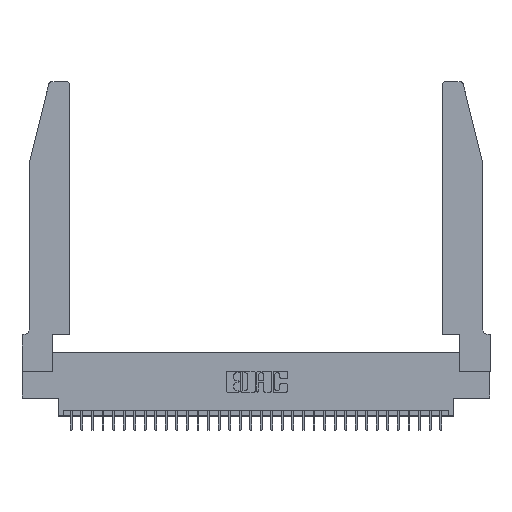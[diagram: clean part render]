
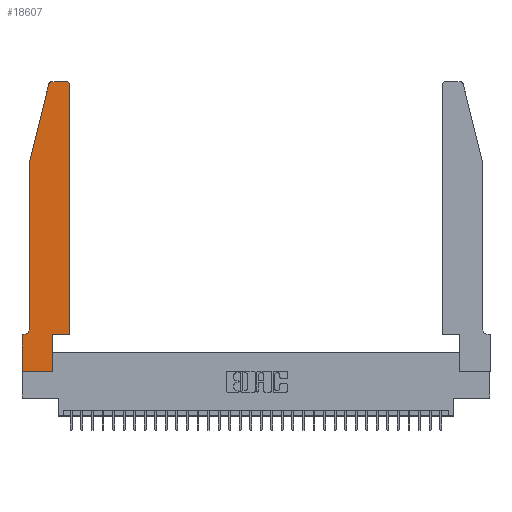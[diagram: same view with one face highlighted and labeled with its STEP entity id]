
A CAD part, top view. The second image highlights one B-rep face of the part: STEP entity #18607.
In plain terms, the highlighted planar face has unit normal (0, 0, 1).
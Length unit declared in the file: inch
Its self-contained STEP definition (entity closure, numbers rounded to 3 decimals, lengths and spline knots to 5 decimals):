
#76 = LINE ( 'NONE', #13323, #6920 ) ;
#954 = DIRECTION ( 'NONE',  ( 0., 1., 0. ) ) ;
#1054 = DIRECTION ( 'NONE',  ( 1., 0., 0. ) ) ;
#1309 = VERTEX_POINT ( 'NONE', #8028 ) ;
#1374 = EDGE_CURVE ( 'NONE', #4359, #28598, #26620, .T. ) ;
#1521 = CARTESIAN_POINT ( 'NONE',  ( 0., 0.35, 0.37 ) ) ;
#1557 = DIRECTION ( 'NONE',  ( 1., 0., 0. ) ) ;
#1675 = DIRECTION ( 'NONE',  ( 0., 0., 1. ) ) ;
#1846 = CARTESIAN_POINT ( 'NONE',  ( 0.2865, 0.35, 0.37 ) ) ;
#2091 = VERTEX_POINT ( 'NONE', #13837 ) ;
#2400 = VERTEX_POINT ( 'NONE', #10340 ) ;
#2531 = DIRECTION ( 'NONE',  ( 0., -1., 0. ) ) ;
#2763 = DIRECTION ( 'NONE',  ( 1., 0., 0. ) ) ;
#3043 = LINE ( 'NONE', #13527, #30806 ) ;
#3999 = AXIS2_PLACEMENT_3D ( 'NONE', #25015, #24501, #30032 ) ;
#4359 = VERTEX_POINT ( 'NONE', #29750 ) ;
#4598 = VECTOR ( 'NONE', #1557, 39.37008 ) ;
#4768 = CARTESIAN_POINT ( 'NONE',  ( 0.25487, 2.72718, 0.37 ) ) ;
#5093 = EDGE_CURVE ( 'NONE', #24850, #13024, #31501, .T. ) ;
#6107 = EDGE_CURVE ( 'NONE', #28598, #2400, #19819, .T. ) ;
#6110 = CARTESIAN_POINT ( 'NONE',  ( 0.2865, 0.35, 0.37 ) ) ;
#6686 = PLANE ( 'NONE',  #24319 ) ;
#6690 = EDGE_CURVE ( 'NONE', #1309, #9084, #20849, .T. ) ;
#6920 = VECTOR ( 'NONE', #24038, 39.37008 ) ;
#7410 = ORIENTED_EDGE ( 'NONE', *, *, #29518, .T. ) ;
#7415 = LINE ( 'NONE', #20180, #26383 ) ;
#7442 = EDGE_LOOP ( 'NONE', ( #7410, #22434, #31348, #13535, #31731, #28482, #27480, #15496, #32855, #11401, #15814, #26457 ) ) ;
#7660 = AXIS2_PLACEMENT_3D ( 'NONE', #24821, #19822, #1054 ) ;
#7762 = CARTESIAN_POINT ( 'NONE',  ( 0., 0., 0.37 ) ) ;
#8028 = CARTESIAN_POINT ( 'NONE',  ( 0., 0.35, 0.37 ) ) ;
#8782 = CARTESIAN_POINT ( 'NONE',  ( 0.4205, 2.72, 0.37 ) ) ;
#9084 = VERTEX_POINT ( 'NONE', #31562 ) ;
#9114 = DIRECTION ( 'NONE',  ( 0., 0., 1. ) ) ;
#9442 = DIRECTION ( 'NONE',  ( 1., 0., 0. ) ) ;
#9764 = EDGE_CURVE ( 'NONE', #28842, #2091, #22382, .T. ) ;
#10015 = LINE ( 'NONE', #20533, #29179 ) ;
#10340 = CARTESIAN_POINT ( 'NONE',  ( 0.4505, 0.35, 0.37 ) ) ;
#10406 = EDGE_CURVE ( 'NONE', #2400, #28842, #76, .T. ) ;
#11153 = VECTOR ( 'NONE', #21382, 39.37008 ) ;
#11401 = ORIENTED_EDGE ( 'NONE', *, *, #6107, .T. ) ;
#11603 = CARTESIAN_POINT ( 'NONE',  ( 0.0755, 0.42, 0.37 ) ) ;
#12979 = EDGE_CURVE ( 'NONE', #16748, #24606, #18082, .T. ) ;
#13024 = VERTEX_POINT ( 'NONE', #30683 ) ;
#13323 = CARTESIAN_POINT ( 'NONE',  ( 0.4505, 0.35, 0.37 ) ) ;
#13527 = CARTESIAN_POINT ( 'NONE',  ( 0.0755, 2., 0.37 ) ) ;
#13535 = ORIENTED_EDGE ( 'NONE', *, *, #13633, .T. ) ;
#13633 = EDGE_CURVE ( 'NONE', #23809, #24850, #3043, .T. ) ;
#13837 = CARTESIAN_POINT ( 'NONE',  ( 0.4205, 2.75, 0.37 ) ) ;
#15496 = ORIENTED_EDGE ( 'NONE', *, *, #16502, .T. ) ;
#15602 = VECTOR ( 'NONE', #23781, 39.37008 ) ;
#15814 = ORIENTED_EDGE ( 'NONE', *, *, #10406, .T. ) ;
#16332 = VECTOR ( 'NONE', #26514, 39.37008 ) ;
#16502 = EDGE_CURVE ( 'NONE', #9084, #4359, #10015, .T. ) ;
#16748 = VERTEX_POINT ( 'NONE', #29151 ) ;
#17347 = FACE_OUTER_BOUND ( 'NONE', #7442, .T. ) ;
#18082 = CIRCLE ( 'NONE', #7660, 0.03 ) ;
#18577 = LINE ( 'NONE', #23589, #16332 ) ;
#18607 = ADVANCED_FACE ( 'NONE', ( #17347 ), #6686, .T. ) ;
#19481 = CARTESIAN_POINT ( 'NONE',  ( 0.4505, 0.35, 0.37 ) ) ;
#19687 = EDGE_CURVE ( 'NONE', #13024, #1309, #28999, .T. ) ;
#19819 = LINE ( 'NONE', #19481, #4598 ) ;
#19822 = DIRECTION ( 'NONE',  ( 0., 0., 1. ) ) ;
#19948 = DIRECTION ( 'NONE',  ( 1., 0., 0. ) ) ;
#20180 = CARTESIAN_POINT ( 'NONE',  ( 0.2605, 2.75, 0.37 ) ) ;
#20533 = CARTESIAN_POINT ( 'NONE',  ( 0., 0., 0.37 ) ) ;
#20849 = LINE ( 'NONE', #7762, #15602 ) ;
#21382 = DIRECTION ( 'NONE',  ( -1., 0., 0. ) ) ;
#22382 = CIRCLE ( 'NONE', #25149, 0.03 ) ;
#22434 = ORIENTED_EDGE ( 'NONE', *, *, #12979, .T. ) ;
#23243 = DIRECTION ( 'NONE',  ( -1., 0., 0. ) ) ;
#23500 = CARTESIAN_POINT ( 'NONE',  ( 0.0755, 2., 0.37 ) ) ;
#23589 = CARTESIAN_POINT ( 'NONE',  ( 0.0755, 2., 0.37 ) ) ;
#23781 = DIRECTION ( 'NONE',  ( 0., -1., 0. ) ) ;
#23809 = VERTEX_POINT ( 'NONE', #23500 ) ;
#24038 = DIRECTION ( 'NONE',  ( 0., 1., 0. ) ) ;
#24319 = AXIS2_PLACEMENT_3D ( 'NONE', #1521, #1675, #19948 ) ;
#24396 = CARTESIAN_POINT ( 'NONE',  ( 0.4505, 2.72, 0.37 ) ) ;
#24501 = DIRECTION ( 'NONE',  ( 0., 0., -1. ) ) ;
#24606 = VERTEX_POINT ( 'NONE', #4768 ) ;
#24821 = CARTESIAN_POINT ( 'NONE',  ( 0.284, 2.72, 0.37 ) ) ;
#24850 = VERTEX_POINT ( 'NONE', #11603 ) ;
#25015 = CARTESIAN_POINT ( 'NONE',  ( 0.0055, 0.42, 0.37 ) ) ;
#25149 = AXIS2_PLACEMENT_3D ( 'NONE', #8782, #9114, #9442 ) ;
#26383 = VECTOR ( 'NONE', #23243, 39.37008 ) ;
#26457 = ORIENTED_EDGE ( 'NONE', *, *, #9764, .T. ) ;
#26514 = DIRECTION ( 'NONE',  ( -0.239, -0.971, 0. ) ) ;
#26620 = LINE ( 'NONE', #6110, #30876 ) ;
#27480 = ORIENTED_EDGE ( 'NONE', *, *, #6690, .T. ) ;
#28261 = EDGE_CURVE ( 'NONE', #24606, #23809, #18577, .T. ) ;
#28482 = ORIENTED_EDGE ( 'NONE', *, *, #19687, .T. ) ;
#28598 = VERTEX_POINT ( 'NONE', #1846 ) ;
#28842 = VERTEX_POINT ( 'NONE', #24396 ) ;
#28999 = LINE ( 'NONE', #32071, #11153 ) ;
#29151 = CARTESIAN_POINT ( 'NONE',  ( 0.284, 2.75, 0.37 ) ) ;
#29179 = VECTOR ( 'NONE', #2763, 39.37008 ) ;
#29518 = EDGE_CURVE ( 'NONE', #2091, #16748, #7415, .T. ) ;
#29750 = CARTESIAN_POINT ( 'NONE',  ( 0.2865, 0., 0.37 ) ) ;
#30032 = DIRECTION ( 'NONE',  ( -1., 0., 0. ) ) ;
#30683 = CARTESIAN_POINT ( 'NONE',  ( 0.0055, 0.35, 0.37 ) ) ;
#30806 = VECTOR ( 'NONE', #2531, 39.37008 ) ;
#30876 = VECTOR ( 'NONE', #954, 39.37008 ) ;
#31348 = ORIENTED_EDGE ( 'NONE', *, *, #28261, .T. ) ;
#31501 = CIRCLE ( 'NONE', #3999, 0.07 ) ;
#31562 = CARTESIAN_POINT ( 'NONE',  ( 0., 0., 0.37 ) ) ;
#31731 = ORIENTED_EDGE ( 'NONE', *, *, #5093, .T. ) ;
#32071 = CARTESIAN_POINT ( 'NONE',  ( 0.0755, 0.35, 0.37 ) ) ;
#32855 = ORIENTED_EDGE ( 'NONE', *, *, #1374, .T. ) ;
